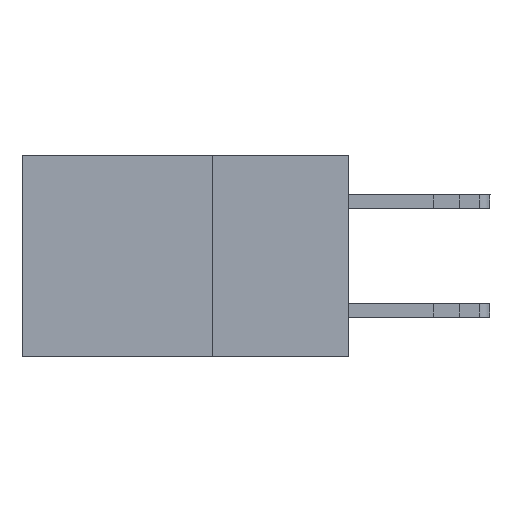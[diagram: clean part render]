
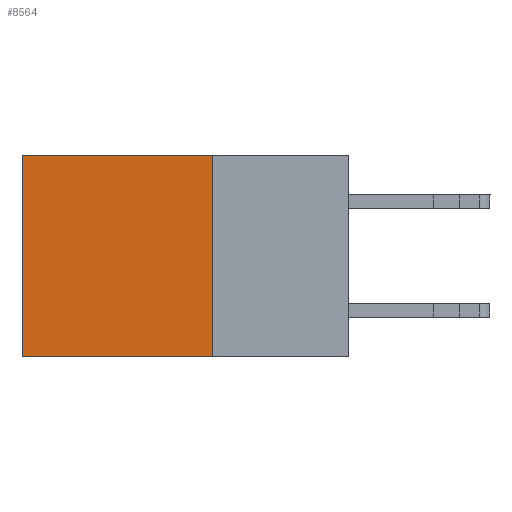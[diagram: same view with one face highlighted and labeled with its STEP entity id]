
A CAD part, left-side view. The second image highlights one B-rep face of the part: STEP entity #8564.
In plain terms, the highlighted planar face has unit normal (-1, 0, 0).
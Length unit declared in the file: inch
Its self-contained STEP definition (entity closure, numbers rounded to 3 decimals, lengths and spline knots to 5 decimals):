
#397 = DIRECTION ( 'NONE',  ( 0., 0., -1. ) ) ;
#1216 = CARTESIAN_POINT ( 'NONE',  ( 0.298, 0.25, -0.37 ) ) ;
#1273 = VERTEX_POINT ( 'NONE', #13490 ) ;
#2367 = VERTEX_POINT ( 'NONE', #6877 ) ;
#2570 = CARTESIAN_POINT ( 'NONE',  ( 0.298, 0.25, 0. ) ) ;
#2910 = LINE ( 'NONE', #11171, #25487 ) ;
#3622 = ORIENTED_EDGE ( 'NONE', *, *, #12570, .T. ) ;
#3625 = ORIENTED_EDGE ( 'NONE', *, *, #22554, .T. ) ;
#5790 = FACE_OUTER_BOUND ( 'NONE', #22088, .T. ) ;
#6877 = CARTESIAN_POINT ( 'NONE',  ( 0.298, 0.25, 0. ) ) ;
#7013 = CARTESIAN_POINT ( 'NONE',  ( 0.298, 0.6, 0. ) ) ;
#7964 = ORIENTED_EDGE ( 'NONE', *, *, #8413, .F. ) ;
#8413 = EDGE_CURVE ( 'NONE', #2367, #9445, #11374, .T. ) ;
#8564 = ADVANCED_FACE ( 'NONE', ( #5790 ), #9724, .F. ) ;
#9135 = DIRECTION ( 'NONE',  ( 0., 1., 0. ) ) ;
#9445 = VERTEX_POINT ( 'NONE', #1216 ) ;
#9724 = PLANE ( 'NONE',  #19551 ) ;
#9768 = VECTOR ( 'NONE', #397, 39.37008 ) ;
#11171 = CARTESIAN_POINT ( 'NONE',  ( 0.298, 0.25, -0.37 ) ) ;
#11374 = LINE ( 'NONE', #2570, #20849 ) ;
#11503 = DIRECTION ( 'NONE',  ( 0., 0., -1. ) ) ;
#11646 = VECTOR ( 'NONE', #17369, 39.37008 ) ;
#11960 = VERTEX_POINT ( 'NONE', #20080 ) ;
#12570 = EDGE_CURVE ( 'NONE', #11960, #1273, #16894, .T. ) ;
#12857 = DIRECTION ( 'NONE',  ( 0., 0., -1. ) ) ;
#13490 = CARTESIAN_POINT ( 'NONE',  ( 0.298, 0.6, -0.37 ) ) ;
#13572 = CARTESIAN_POINT ( 'NONE',  ( 0.298, 0.25, 0. ) ) ;
#13768 = CARTESIAN_POINT ( 'NONE',  ( 0.298, 0.25, 0. ) ) ;
#16894 = LINE ( 'NONE', #7013, #9768 ) ;
#17369 = DIRECTION ( 'NONE',  ( 0., 1., 0. ) ) ;
#19551 = AXIS2_PLACEMENT_3D ( 'NONE', #13768, #22033, #11503 ) ;
#20080 = CARTESIAN_POINT ( 'NONE',  ( 0.298, 0.6, 0. ) ) ;
#20849 = VECTOR ( 'NONE', #12857, 39.37008 ) ;
#22033 = DIRECTION ( 'NONE',  ( 1., 0., 0. ) ) ;
#22088 = EDGE_LOOP ( 'NONE', ( #3622, #23042, #7964, #3625 ) ) ;
#22554 = EDGE_CURVE ( 'NONE', #2367, #11960, #23732, .T. ) ;
#23042 = ORIENTED_EDGE ( 'NONE', *, *, #25756, .F. ) ;
#23732 = LINE ( 'NONE', #13572, #11646 ) ;
#25487 = VECTOR ( 'NONE', #9135, 39.37008 ) ;
#25756 = EDGE_CURVE ( 'NONE', #9445, #1273, #2910, .T. ) ;
